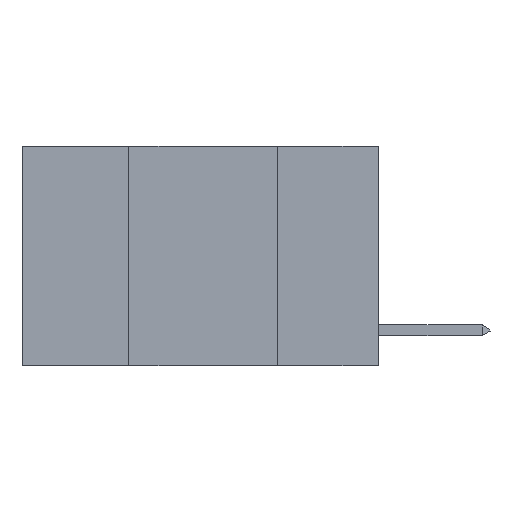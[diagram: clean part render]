
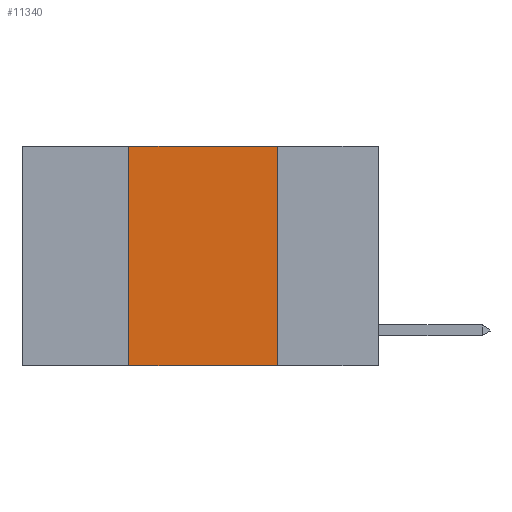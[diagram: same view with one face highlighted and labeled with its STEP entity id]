
A CAD part, left-side view. The second image highlights one B-rep face of the part: STEP entity #11340.
In plain terms, the highlighted planar face has unit normal (-1, 0, 0).
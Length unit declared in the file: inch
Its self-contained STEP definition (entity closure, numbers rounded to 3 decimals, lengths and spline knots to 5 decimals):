
#180 = VECTOR ( 'NONE', #4754, 39.37008 ) ;
#347 = PLANE ( 'NONE',  #12680 ) ;
#423 = CARTESIAN_POINT ( 'NONE',  ( 0., 0.17, 0. ) ) ;
#542 = LINE ( 'NONE', #423, #180 ) ;
#671 = EDGE_CURVE ( 'NONE', #7873, #7867, #6355, .T. ) ;
#810 = DIRECTION ( 'NONE',  ( 0., 0., 1. ) ) ;
#1545 = EDGE_CURVE ( 'NONE', #7873, #10333, #5346, .T. ) ;
#1839 = DIRECTION ( 'NONE',  ( 0., -1., 0. ) ) ;
#1955 = CARTESIAN_POINT ( 'NONE',  ( 0., 0.6, -0.37 ) ) ;
#2145 = EDGE_LOOP ( 'NONE', ( #12290, #10732, #10844, #6926 ) ) ;
#2491 = CARTESIAN_POINT ( 'NONE',  ( 0., 0.42, 0. ) ) ;
#2512 = VECTOR ( 'NONE', #11647, 39.37008 ) ;
#2577 = DIRECTION ( 'NONE',  ( 1., 0., 0. ) ) ;
#2587 = CARTESIAN_POINT ( 'NONE',  ( 0., 0.42, 0. ) ) ;
#3264 = VECTOR ( 'NONE', #810, 39.37008 ) ;
#3437 = VERTEX_POINT ( 'NONE', #8495 ) ;
#3781 = EDGE_CURVE ( 'NONE', #3437, #10333, #542, .T. ) ;
#4376 = LINE ( 'NONE', #5085, #12857 ) ;
#4534 = FACE_OUTER_BOUND ( 'NONE', #2145, .T. ) ;
#4754 = DIRECTION ( 'NONE',  ( 0., 0., -1. ) ) ;
#5085 = CARTESIAN_POINT ( 'NONE',  ( 0., 0.6, 0. ) ) ;
#5346 = LINE ( 'NONE', #1955, #2512 ) ;
#6252 = CARTESIAN_POINT ( 'NONE',  ( 0., 0.17, -0.37 ) ) ;
#6355 = LINE ( 'NONE', #2587, #3264 ) ;
#6774 = CARTESIAN_POINT ( 'NONE',  ( 0., 0.6, 0. ) ) ;
#6926 = ORIENTED_EDGE ( 'NONE', *, *, #1545, .T. ) ;
#7867 = VERTEX_POINT ( 'NONE', #2491 ) ;
#7873 = VERTEX_POINT ( 'NONE', #9909 ) ;
#8495 = CARTESIAN_POINT ( 'NONE',  ( 0., 0.17, 0. ) ) ;
#9909 = CARTESIAN_POINT ( 'NONE',  ( 0., 0.42, -0.37 ) ) ;
#10000 = DIRECTION ( 'NONE',  ( 0., 0., -1. ) ) ;
#10333 = VERTEX_POINT ( 'NONE', #6252 ) ;
#10732 = ORIENTED_EDGE ( 'NONE', *, *, #11579, .F. ) ;
#10844 = ORIENTED_EDGE ( 'NONE', *, *, #671, .F. ) ;
#11340 = ADVANCED_FACE ( 'NONE', ( #4534 ), #347, .F. ) ;
#11579 = EDGE_CURVE ( 'NONE', #7867, #3437, #4376, .T. ) ;
#11647 = DIRECTION ( 'NONE',  ( 0., -1., 0. ) ) ;
#12290 = ORIENTED_EDGE ( 'NONE', *, *, #3781, .F. ) ;
#12680 = AXIS2_PLACEMENT_3D ( 'NONE', #6774, #2577, #10000 ) ;
#12857 = VECTOR ( 'NONE', #1839, 39.37008 ) ;
